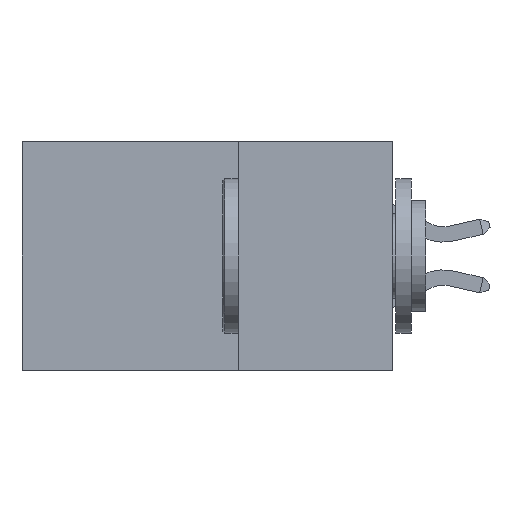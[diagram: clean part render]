
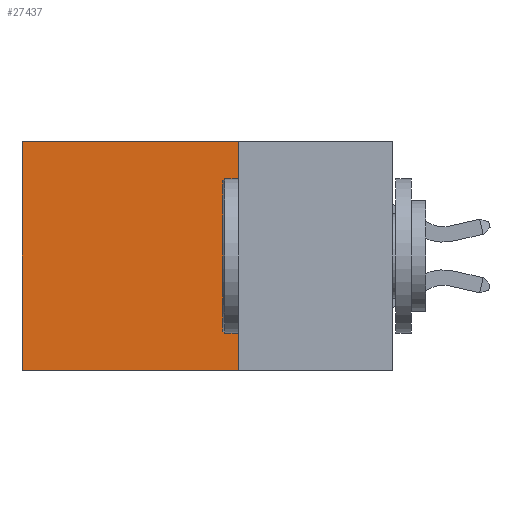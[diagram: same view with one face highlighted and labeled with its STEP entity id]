
A CAD part, left-side view. The second image highlights one B-rep face of the part: STEP entity #27437.
In plain terms, the highlighted planar face has unit normal (-1, 0, 0).
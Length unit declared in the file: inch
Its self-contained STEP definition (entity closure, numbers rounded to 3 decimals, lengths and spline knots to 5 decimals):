
#579 = VECTOR ( 'NONE', #31565, 39.37008 ) ;
#683 = VECTOR ( 'NONE', #7827, 39.37008 ) ;
#1575 = ORIENTED_EDGE ( 'NONE', *, *, #13129, .T. ) ;
#7606 = ORIENTED_EDGE ( 'NONE', *, *, #30937, .F. ) ;
#7827 = DIRECTION ( 'NONE',  ( 0., 1., 0. ) ) ;
#7908 = LINE ( 'NONE', #21115, #683 ) ;
#9815 = CARTESIAN_POINT ( 'NONE',  ( 0.2875, 0.25, 0. ) ) ;
#9965 = CARTESIAN_POINT ( 'NONE',  ( 0.2875, 0.25, -0.37 ) ) ;
#10924 = CARTESIAN_POINT ( 'NONE',  ( 0.2875, 0.25, 0. ) ) ;
#11050 = EDGE_CURVE ( 'NONE', #12364, #15941, #7908, .T. ) ;
#11143 = VERTEX_POINT ( 'NONE', #24004 ) ;
#12295 = ORIENTED_EDGE ( 'NONE', *, *, #11050, .F. ) ;
#12364 = VERTEX_POINT ( 'NONE', #9965 ) ;
#12465 = DIRECTION ( 'NONE',  ( 1., 0., 0. ) ) ;
#13129 = EDGE_CURVE ( 'NONE', #20387, #15941, #21162, .T. ) ;
#15084 = CARTESIAN_POINT ( 'NONE',  ( 0.2875, 0.25, 0. ) ) ;
#15941 = VERTEX_POINT ( 'NONE', #30539 ) ;
#15969 = LINE ( 'NONE', #15084, #29280 ) ;
#17765 = DIRECTION ( 'NONE',  ( 0., 0., -1. ) ) ;
#20387 = VERTEX_POINT ( 'NONE', #32419 ) ;
#21115 = CARTESIAN_POINT ( 'NONE',  ( 0.2875, 0.25, -0.37 ) ) ;
#21162 = LINE ( 'NONE', #28946, #579 ) ;
#22906 = FACE_OUTER_BOUND ( 'NONE', #32110, .T. ) ;
#23738 = LINE ( 'NONE', #10924, #29904 ) ;
#24004 = CARTESIAN_POINT ( 'NONE',  ( 0.2875, 0.25, 0. ) ) ;
#25620 = ORIENTED_EDGE ( 'NONE', *, *, #28079, .T. ) ;
#25761 = PLANE ( 'NONE',  #29828 ) ;
#27437 = ADVANCED_FACE ( 'NONE', ( #22906 ), #25761, .F. ) ;
#28079 = EDGE_CURVE ( 'NONE', #11143, #20387, #23738, .T. ) ;
#28946 = CARTESIAN_POINT ( 'NONE',  ( 0.2875, 0.6, 0. ) ) ;
#29280 = VECTOR ( 'NONE', #17765, 39.37008 ) ;
#29828 = AXIS2_PLACEMENT_3D ( 'NONE', #9815, #12465, #30996 ) ;
#29904 = VECTOR ( 'NONE', #32108, 39.37008 ) ;
#30539 = CARTESIAN_POINT ( 'NONE',  ( 0.2875, 0.6, -0.37 ) ) ;
#30937 = EDGE_CURVE ( 'NONE', #11143, #12364, #15969, .T. ) ;
#30996 = DIRECTION ( 'NONE',  ( 0., 0., -1. ) ) ;
#31565 = DIRECTION ( 'NONE',  ( 0., 0., -1. ) ) ;
#32108 = DIRECTION ( 'NONE',  ( 0., 1., 0. ) ) ;
#32110 = EDGE_LOOP ( 'NONE', ( #1575, #12295, #7606, #25620 ) ) ;
#32419 = CARTESIAN_POINT ( 'NONE',  ( 0.2875, 0.6, 0. ) ) ;
